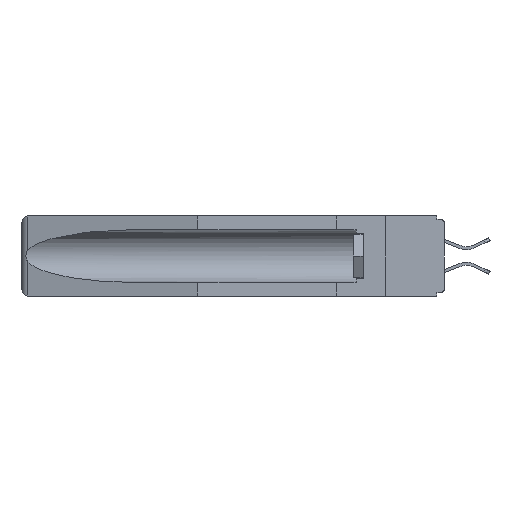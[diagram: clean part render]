
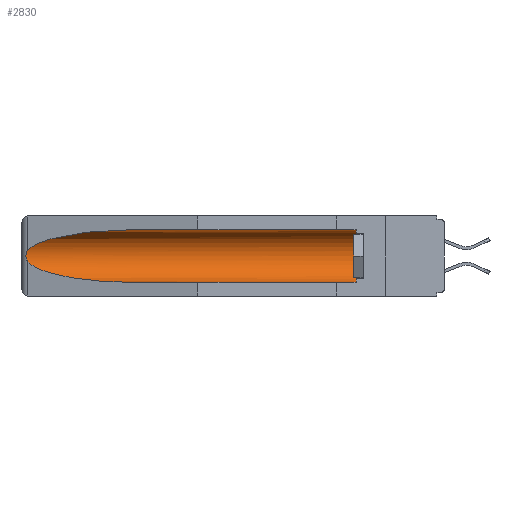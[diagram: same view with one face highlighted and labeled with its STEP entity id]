
A CAD part, left-side view. The second image highlights one B-rep face of the part: STEP entity #2830.
In plain terms, the highlighted cylindrical face has radius 2.857 mm (diameter 5.715 mm), a partial arc.
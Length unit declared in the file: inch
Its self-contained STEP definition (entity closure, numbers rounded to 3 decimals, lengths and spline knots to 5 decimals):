
#41 = VERTEX_POINT ( 'NONE', #2524 ) ;
#125 = EDGE_CURVE ( 'NONE', #15544, #2202, #23208, .T. ) ;
#178 = VERTEX_POINT ( 'NONE', #1479 ) ;
#192 = CARTESIAN_POINT ( 'NONE',  ( 0.25451, 1.48313, -0.24835 ) ) ;
#401 = ORIENTED_EDGE ( 'NONE', *, *, #125, .F. ) ;
#728 = EDGE_CURVE ( 'NONE', #41, #3907, #6069, .T. ) ;
#1479 = CARTESIAN_POINT ( 'NONE',  ( 0.155, 1.07973, -0.059 ) ) ;
#1523 = CARTESIAN_POINT ( 'NONE',  ( 0.155, 0.126, -0.284 ) ) ;
#2202 = VERTEX_POINT ( 'NONE', #10992 ) ;
#2524 = CARTESIAN_POINT ( 'NONE',  ( 0.26537, 1.52718, -0.14972 ) ) ;
#2830 = ADVANCED_FACE ( 'NONE', ( #4703 ), #21011, .F. ) ;
#3094 = CARTESIAN_POINT ( 'NONE',  ( 0.2673, 1.53269, -0.17917 ) ) ;
#3907 = VERTEX_POINT ( 'NONE', #9888 ) ;
#3997 = CARTESIAN_POINT ( 'NONE',  ( 0.26537, 1.52718, -0.19328 ) ) ;
#4110 = ORIENTED_EDGE ( 'NONE', *, *, #728, .T. ) ;
#4635 = DIRECTION ( 'NONE',  ( 0., 0., 1. ) ) ;
#4703 = FACE_OUTER_BOUND ( 'NONE', #11881, .T. ) ;
#4825 = ORIENTED_EDGE ( 'NONE', *, *, #14609, .T. ) ;
#4955 = CARTESIAN_POINT ( 'NONE',  ( 0.2673, 1.5327, -0.16383 ) ) ;
#6069 = B_SPLINE_CURVE_WITH_KNOTS ( 'NONE', 3,
 ( #10665, #8656, #23824, #4955, #16117, #19852, #3094, #14215, #10581, #8739 ),
 .UNSPECIFIED., .F., .F.,
 ( 4, 2, 2, 2, 4 ),
 ( 0., 0.00029, 0.00058, 0.00087, 0.00117 ),
 .UNSPECIFIED. ) ;
#7042 = DIRECTION ( 'NONE',  ( 0., 0., 1. ) ) ;
#7239 = VECTOR ( 'NONE', #8817, 39.37008 ) ;
#7422 = CARTESIAN_POINT ( 'NONE',  ( 0.155, 1.07973, -0.284 ) ) ;
#8154 = CARTESIAN_POINT ( 'NONE',  ( 0.155, 0.126, -0.059 ) ) ;
#8656 = CARTESIAN_POINT ( 'NONE',  ( 0.26597, 1.52961, -0.15275 ) ) ;
#8739 = CARTESIAN_POINT ( 'NONE',  ( 0.26537, 1.52718, -0.19328 ) ) ;
#8817 = DIRECTION ( 'NONE',  ( 0., 1., 0. ) ) ;
#9865 = LINE ( 'NONE', #12491, #7239 ) ;
#9888 = CARTESIAN_POINT ( 'NONE',  ( 0.26537, 1.52718, -0.19328 ) ) ;
#10581 = CARTESIAN_POINT ( 'NONE',  ( 0.26597, 1.5296, -0.19026 ) ) ;
#10665 = CARTESIAN_POINT ( 'NONE',  ( 0.26537, 1.52718, -0.14972 ) ) ;
#10992 = CARTESIAN_POINT ( 'NONE',  ( 0.155, 1.07973, -0.284 ) ) ;
#11881 = EDGE_LOOP ( 'NONE', ( #21783, #4110, #16243, #401, #17595, #4825 ) ) ;
#12054 = CARTESIAN_POINT ( 'NONE',  ( 0.21114, 1.30732, -0.059 ) ) ;
#12327 = DIRECTION ( 'NONE',  ( 0., 1., 0. ) ) ;
#12491 = CARTESIAN_POINT ( 'NONE',  ( 0.155, -0.30754, -0.059 ) ) ;
#13172 = CARTESIAN_POINT ( 'NONE',  ( 0.21114, 1.30732, -0.284 ) ) ;
#13557 = AXIS2_PLACEMENT_3D ( 'NONE', #17391, #16013, #4635 ) ;
#13912 = CARTESIAN_POINT ( 'NONE',  ( 0.25451, 1.48313, -0.09465 ) ) ;
#14118 =( BOUNDED_CURVE ( )  B_SPLINE_CURVE ( 3, ( #3997, #192, #13172, #7422 ),
 .UNSPECIFIED., .F., .F. ) 
 B_SPLINE_CURVE_WITH_KNOTS ( ( 4, 4 ),
 ( 0.1948, 1.5708 ),
 .UNSPECIFIED. ) 
 CURVE ( )  GEOMETRIC_REPRESENTATION_ITEM ( )  RATIONAL_B_SPLINE_CURVE ( ( 1., 0.848, 0.848, 1. ) ) 
 REPRESENTATION_ITEM ( '' )  );
#14215 = CARTESIAN_POINT ( 'NONE',  ( 0.26655, 1.53094, -0.18657 ) ) ;
#14609 = EDGE_CURVE ( 'NONE', #19194, #178, #9865, .T. ) ;
#15544 = VERTEX_POINT ( 'NONE', #1523 ) ;
#15586 = EDGE_CURVE ( 'NONE', #3907, #2202, #14118, .T. ) ;
#15918 = DIRECTION ( 'NONE',  ( 0., 1., 0. ) ) ;
#16013 = DIRECTION ( 'NONE',  ( 0., -1., 0. ) ) ;
#16117 = CARTESIAN_POINT ( 'NONE',  ( 0.2675, 1.53308, -0.16763 ) ) ;
#16243 = ORIENTED_EDGE ( 'NONE', *, *, #15586, .T. ) ;
#16266 = AXIS2_PLACEMENT_3D ( 'NONE', #23294, #15918, #7042 ) ;
#17391 = CARTESIAN_POINT ( 'NONE',  ( 0.155, 0.126, -0.1715 ) ) ;
#17595 = ORIENTED_EDGE ( 'NONE', *, *, #22934, .T. ) ;
#17942 = EDGE_CURVE ( 'NONE', #178, #41, #18743, .T. ) ;
#18743 =( BOUNDED_CURVE ( )  B_SPLINE_CURVE ( 3, ( #19464, #12054, #13912, #23044 ),
 .UNSPECIFIED., .F., .T. ) 
 B_SPLINE_CURVE_WITH_KNOTS ( ( 4, 4 ),
 ( 4.71239, 6.08839 ),
 .UNSPECIFIED. ) 
 CURVE ( )  GEOMETRIC_REPRESENTATION_ITEM ( )  RATIONAL_B_SPLINE_CURVE ( ( 1., 0.848, 0.848, 1. ) ) 
 REPRESENTATION_ITEM ( '' )  );
#19194 = VERTEX_POINT ( 'NONE', #8154 ) ;
#19464 = CARTESIAN_POINT ( 'NONE',  ( 0.155, 1.07973, -0.059 ) ) ;
#19598 = CIRCLE ( 'NONE', #13557, 0.1125 ) ;
#19852 = CARTESIAN_POINT ( 'NONE',  ( 0.2675, 1.53308, -0.17534 ) ) ;
#21011 = CYLINDRICAL_SURFACE ( 'NONE', #16266, 0.1125 ) ;
#21729 = VECTOR ( 'NONE', #12327, 39.37008 ) ;
#21783 = ORIENTED_EDGE ( 'NONE', *, *, #17942, .T. ) ;
#22934 = EDGE_CURVE ( 'NONE', #15544, #19194, #19598, .T. ) ;
#23044 = CARTESIAN_POINT ( 'NONE',  ( 0.26537, 1.52718, -0.14972 ) ) ;
#23208 = LINE ( 'NONE', #23488, #21729 ) ;
#23294 = CARTESIAN_POINT ( 'NONE',  ( 0.155, -0.30754, -0.1715 ) ) ;
#23488 = CARTESIAN_POINT ( 'NONE',  ( 0.155, -0.30754, -0.284 ) ) ;
#23824 = CARTESIAN_POINT ( 'NONE',  ( 0.26654, 1.53092, -0.15636 ) ) ;
